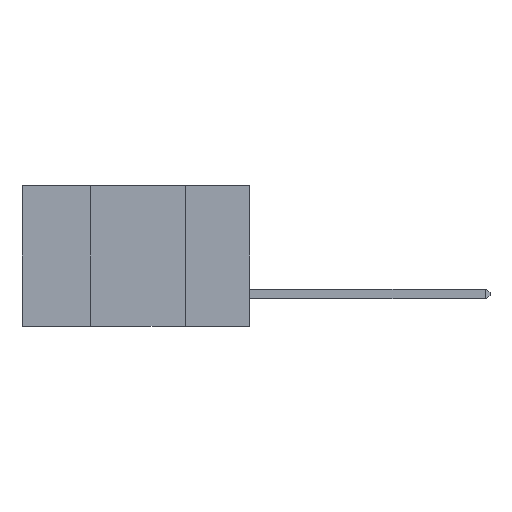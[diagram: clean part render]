
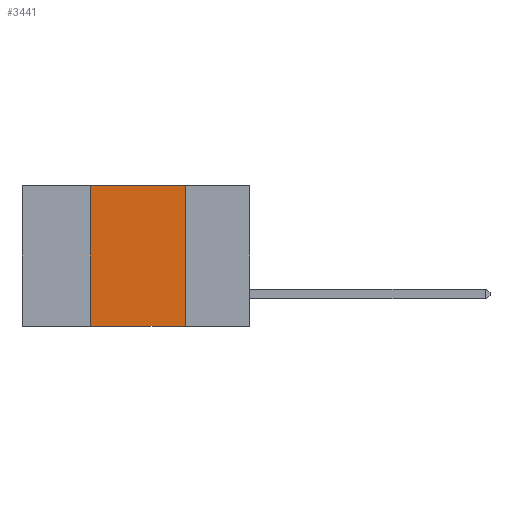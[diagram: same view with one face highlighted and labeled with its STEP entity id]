
A CAD part, left-side view. The second image highlights one B-rep face of the part: STEP entity #3441.
In plain terms, the highlighted planar face has unit normal (-1, 0, 0).
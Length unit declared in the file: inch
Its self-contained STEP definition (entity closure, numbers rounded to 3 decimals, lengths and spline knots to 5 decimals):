
#6 = ORIENTED_EDGE ( 'NONE', *, *, #3562, .F. ) ;
#504 = CARTESIAN_POINT ( 'NONE',  ( 0., 0.6, 0. ) ) ;
#785 = CARTESIAN_POINT ( 'NONE',  ( 0., 0.6, 0. ) ) ;
#814 = VERTEX_POINT ( 'NONE', #8734 ) ;
#880 = ORIENTED_EDGE ( 'NONE', *, *, #7981, .T. ) ;
#988 = CARTESIAN_POINT ( 'NONE',  ( 0., 0.42, 0. ) ) ;
#1194 = ORIENTED_EDGE ( 'NONE', *, *, #6287, .F. ) ;
#1399 = AXIS2_PLACEMENT_3D ( 'NONE', #504, #1445, #1908 ) ;
#1445 = DIRECTION ( 'NONE',  ( 1., 0., 0. ) ) ;
#1658 = VECTOR ( 'NONE', #8597, 39.37008 ) ;
#1908 = DIRECTION ( 'NONE',  ( 0., 0., -1. ) ) ;
#1934 = VERTEX_POINT ( 'NONE', #2249 ) ;
#1959 = VERTEX_POINT ( 'NONE', #6126 ) ;
#2249 = CARTESIAN_POINT ( 'NONE',  ( 0., 0.17, -0.37 ) ) ;
#3021 = EDGE_LOOP ( 'NONE', ( #1194, #3022, #6, #880 ) ) ;
#3022 = ORIENTED_EDGE ( 'NONE', *, *, #9421, .F. ) ;
#3316 = DIRECTION ( 'NONE',  ( 0., -1., 0. ) ) ;
#3441 = ADVANCED_FACE ( 'NONE', ( #8364 ), #4129, .F. ) ;
#3454 = CARTESIAN_POINT ( 'NONE',  ( 0., 0.17, 0. ) ) ;
#3562 = EDGE_CURVE ( 'NONE', #814, #1959, #5176, .T. ) ;
#4129 = PLANE ( 'NONE',  #1399 ) ;
#5176 = LINE ( 'NONE', #988, #9086 ) ;
#6126 = CARTESIAN_POINT ( 'NONE',  ( 0., 0.42, 0. ) ) ;
#6287 = EDGE_CURVE ( 'NONE', #7136, #1934, #9774, .T. ) ;
#6488 = LINE ( 'NONE', #9699, #8441 ) ;
#7136 = VERTEX_POINT ( 'NONE', #3454 ) ;
#7878 = VECTOR ( 'NONE', #3316, 39.37008 ) ;
#7981 = EDGE_CURVE ( 'NONE', #814, #1934, #6488, .T. ) ;
#8089 = LINE ( 'NONE', #785, #7878 ) ;
#8364 = FACE_OUTER_BOUND ( 'NONE', #3021, .T. ) ;
#8441 = VECTOR ( 'NONE', #9728, 39.37008 ) ;
#8597 = DIRECTION ( 'NONE',  ( 0., 0., -1. ) ) ;
#8734 = CARTESIAN_POINT ( 'NONE',  ( 0., 0.42, -0.37 ) ) ;
#9086 = VECTOR ( 'NONE', #9202, 39.37008 ) ;
#9202 = DIRECTION ( 'NONE',  ( 0., 0., 1. ) ) ;
#9225 = CARTESIAN_POINT ( 'NONE',  ( 0., 0.17, 0. ) ) ;
#9421 = EDGE_CURVE ( 'NONE', #1959, #7136, #8089, .T. ) ;
#9699 = CARTESIAN_POINT ( 'NONE',  ( 0., 0.6, -0.37 ) ) ;
#9728 = DIRECTION ( 'NONE',  ( 0., -1., 0. ) ) ;
#9774 = LINE ( 'NONE', #9225, #1658 ) ;
